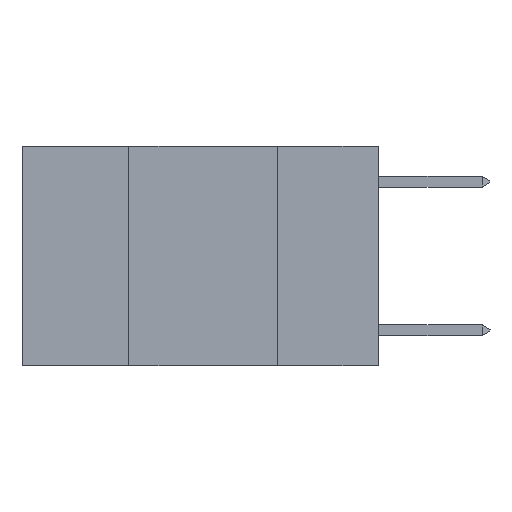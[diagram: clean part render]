
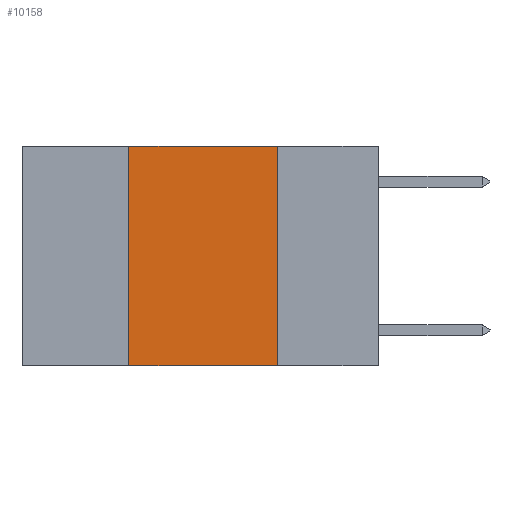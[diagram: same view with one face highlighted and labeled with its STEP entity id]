
A CAD part, left-side view. The second image highlights one B-rep face of the part: STEP entity #10158.
In plain terms, the highlighted planar face has unit normal (-1, 0, 0).
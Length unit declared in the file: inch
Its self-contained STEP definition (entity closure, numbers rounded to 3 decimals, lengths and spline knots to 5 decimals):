
#183 = DIRECTION ( 'NONE',  ( 0., -1., 0. ) ) ;
#613 = DIRECTION ( 'NONE',  ( 1., 0., 0. ) ) ;
#836 = EDGE_CURVE ( 'NONE', #4018, #9006, #1361, .T. ) ;
#882 = VECTOR ( 'NONE', #13538, 39.37008 ) ;
#1296 = EDGE_CURVE ( 'NONE', #7161, #2575, #3865, .T. ) ;
#1320 = VECTOR ( 'NONE', #11815, 39.37008 ) ;
#1361 = LINE ( 'NONE', #7367, #9836 ) ;
#1700 = EDGE_LOOP ( 'NONE', ( #3749, #3238, #8432, #13949 ) ) ;
#1773 = CARTESIAN_POINT ( 'NONE',  ( 0., 0.42, 0. ) ) ;
#2575 = VERTEX_POINT ( 'NONE', #12949 ) ;
#3238 = ORIENTED_EDGE ( 'NONE', *, *, #6122, .F. ) ;
#3749 = ORIENTED_EDGE ( 'NONE', *, *, #1296, .F. ) ;
#3865 = LINE ( 'NONE', #14130, #882 ) ;
#4018 = VERTEX_POINT ( 'NONE', #10998 ) ;
#4305 = LINE ( 'NONE', #5352, #1320 ) ;
#4537 = FACE_OUTER_BOUND ( 'NONE', #1700, .T. ) ;
#5094 = PLANE ( 'NONE',  #7560 ) ;
#5352 = CARTESIAN_POINT ( 'NONE',  ( 0., 0.6, -0.37 ) ) ;
#5483 = DIRECTION ( 'NONE',  ( 0., 0., 1. ) ) ;
#6122 = EDGE_CURVE ( 'NONE', #9006, #7161, #9576, .T. ) ;
#6327 = VECTOR ( 'NONE', #183, 39.37008 ) ;
#6540 = CARTESIAN_POINT ( 'NONE',  ( 0., 0.17, 0. ) ) ;
#7161 = VERTEX_POINT ( 'NONE', #6540 ) ;
#7273 = CARTESIAN_POINT ( 'NONE',  ( 0., 0.6, 0. ) ) ;
#7367 = CARTESIAN_POINT ( 'NONE',  ( 0., 0.42, 0. ) ) ;
#7560 = AXIS2_PLACEMENT_3D ( 'NONE', #7273, #613, #8392 ) ;
#8392 = DIRECTION ( 'NONE',  ( 0., 0., -1. ) ) ;
#8432 = ORIENTED_EDGE ( 'NONE', *, *, #836, .F. ) ;
#9006 = VERTEX_POINT ( 'NONE', #1773 ) ;
#9576 = LINE ( 'NONE', #13334, #6327 ) ;
#9836 = VECTOR ( 'NONE', #5483, 39.37008 ) ;
#10158 = ADVANCED_FACE ( 'NONE', ( #4537 ), #5094, .F. ) ;
#10998 = CARTESIAN_POINT ( 'NONE',  ( 0., 0.42, -0.37 ) ) ;
#11815 = DIRECTION ( 'NONE',  ( 0., -1., 0. ) ) ;
#12423 = EDGE_CURVE ( 'NONE', #4018, #2575, #4305, .T. ) ;
#12949 = CARTESIAN_POINT ( 'NONE',  ( 0., 0.17, -0.37 ) ) ;
#13334 = CARTESIAN_POINT ( 'NONE',  ( 0., 0.6, 0. ) ) ;
#13538 = DIRECTION ( 'NONE',  ( 0., 0., -1. ) ) ;
#13949 = ORIENTED_EDGE ( 'NONE', *, *, #12423, .T. ) ;
#14130 = CARTESIAN_POINT ( 'NONE',  ( 0., 0.17, 0. ) ) ;
